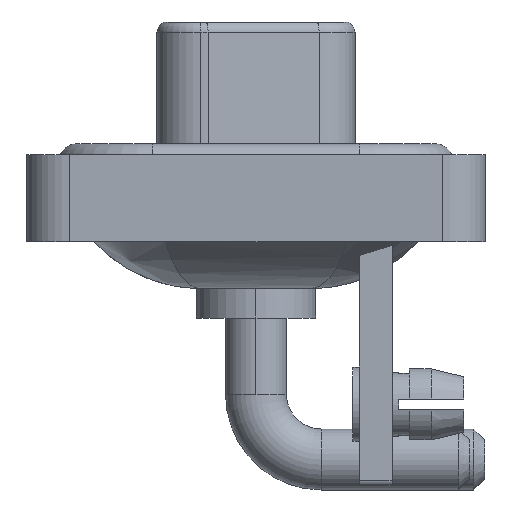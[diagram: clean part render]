
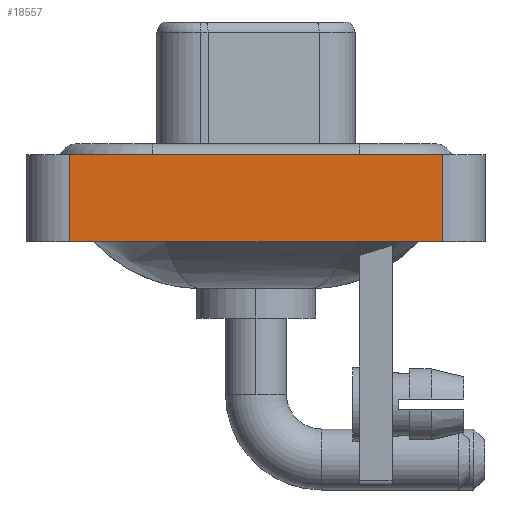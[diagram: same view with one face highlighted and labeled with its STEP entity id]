
A CAD part, left-side view. The second image highlights one B-rep face of the part: STEP entity #18557.
In plain terms, the highlighted planar face has unit normal (-1, 0, 0).
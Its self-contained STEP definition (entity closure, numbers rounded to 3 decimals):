
#1582 = VERTEX_POINT ( 'NONE', #9825 ) ;
#2379 = EDGE_CURVE ( 'NONE', #3491, #17927, #7644, .T. ) ;
#2769 = ORIENTED_EDGE ( 'NONE', *, *, #10308, .T. ) ;
#3050 = EDGE_CURVE ( 'NONE', #4106, #17927, #15314, .T. ) ;
#3079 = CARTESIAN_POINT ( 'NONE',  ( -7.3, -8.55, -3.6 ) ) ;
#3153 = CARTESIAN_POINT ( 'NONE',  ( -7.3, -8.55, -3.6 ) ) ;
#3314 = CARTESIAN_POINT ( 'NONE',  ( -7.3, 8.55, -3.6 ) ) ;
#3491 = VERTEX_POINT ( 'NONE', #16493 ) ;
#3570 = DIRECTION ( 'NONE',  ( 0., 0., 1. ) ) ;
#4106 = VERTEX_POINT ( 'NONE', #15773 ) ;
#4413 = ORIENTED_EDGE ( 'NONE', *, *, #2379, .F. ) ;
#5477 = VECTOR ( 'NONE', #19851, 1000. ) ;
#6748 = VECTOR ( 'NONE', #21480, 1000. ) ;
#7644 = LINE ( 'NONE', #17862, #6748 ) ;
#8235 = LINE ( 'NONE', #3314, #10193 ) ;
#9392 = ORIENTED_EDGE ( 'NONE', *, *, #3050, .T. ) ;
#9825 = CARTESIAN_POINT ( 'NONE',  ( -7.3, 8.55, -3.6 ) ) ;
#9837 = DIRECTION ( 'NONE',  ( -1., 0., 0. ) ) ;
#10193 = VECTOR ( 'NONE', #14827, 1000. ) ;
#10308 = EDGE_CURVE ( 'NONE', #1582, #4106, #12718, .T. ) ;
#11475 = FACE_OUTER_BOUND ( 'NONE', #20960, .T. ) ;
#12718 = LINE ( 'NONE', #3079, #5477 ) ;
#14350 = CARTESIAN_POINT ( 'NONE',  ( -7.3, -8.55, 0.4 ) ) ;
#14827 = DIRECTION ( 'NONE',  ( 0., 0., 1. ) ) ;
#15101 = CARTESIAN_POINT ( 'NONE',  ( -7.3, -8.55, -3.6 ) ) ;
#15314 = LINE ( 'NONE', #15101, #18706 ) ;
#15773 = CARTESIAN_POINT ( 'NONE',  ( -7.3, -8.55, -3.6 ) ) ;
#15863 = DIRECTION ( 'NONE',  ( 0., 0., 1. ) ) ;
#16283 = ORIENTED_EDGE ( 'NONE', *, *, #16320, .F. ) ;
#16320 = EDGE_CURVE ( 'NONE', #1582, #3491, #8235, .T. ) ;
#16493 = CARTESIAN_POINT ( 'NONE',  ( -7.3, 8.55, 0.4 ) ) ;
#17862 = CARTESIAN_POINT ( 'NONE',  ( -7.3, -8.55, 0.4 ) ) ;
#17927 = VERTEX_POINT ( 'NONE', #14350 ) ;
#18176 = PLANE ( 'NONE',  #21426 ) ;
#18557 = ADVANCED_FACE ( 'NONE', ( #11475 ), #18176, .T. ) ;
#18706 = VECTOR ( 'NONE', #3570, 1000. ) ;
#19851 = DIRECTION ( 'NONE',  ( 0., -1., 0. ) ) ;
#20960 = EDGE_LOOP ( 'NONE', ( #9392, #4413, #16283, #2769 ) ) ;
#21426 = AXIS2_PLACEMENT_3D ( 'NONE', #3153, #9837, #15863 ) ;
#21480 = DIRECTION ( 'NONE',  ( 0., -1., 0. ) ) ;
